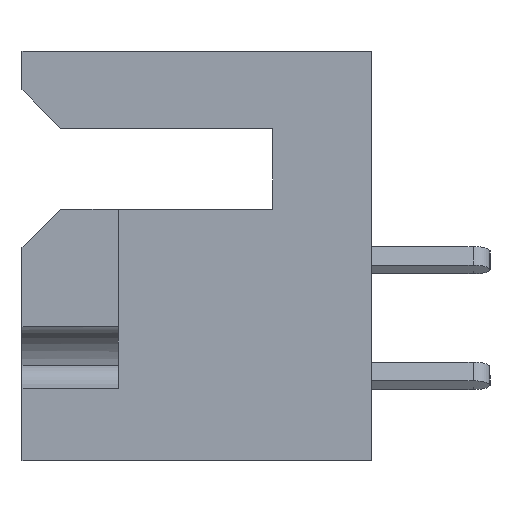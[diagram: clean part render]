
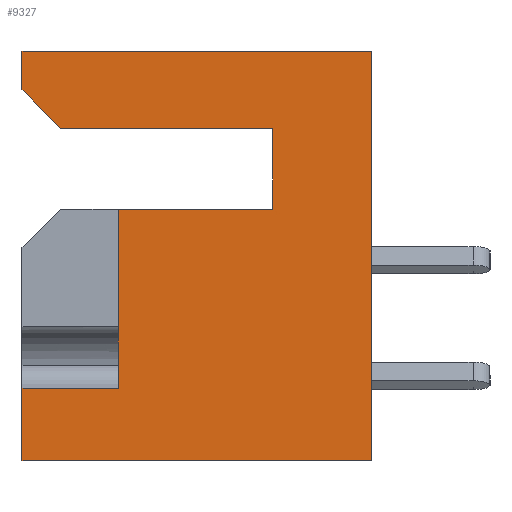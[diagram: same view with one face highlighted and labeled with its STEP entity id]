
A CAD part, left-side view. The second image highlights one B-rep face of the part: STEP entity #9327.
In plain terms, the highlighted planar face has unit normal (-1, 0, 0).
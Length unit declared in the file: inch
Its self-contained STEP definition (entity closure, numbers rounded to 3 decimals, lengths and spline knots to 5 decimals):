
#582 = DIRECTION ( 'NONE',  ( 0., 0., -1. ) ) ;
#656 = DIRECTION ( 'NONE',  ( 0., 0., 1. ) ) ;
#720 = EDGE_LOOP ( 'NONE', ( #2321, #5784, #2436, #14988, #20665, #20450, #15149, #14483, #7558, #4252, #10557 ) ) ;
#765 = VERTEX_POINT ( 'NONE', #15995 ) ;
#1047 = DIRECTION ( 'NONE',  ( 0., 0., 1. ) ) ;
#1205 = VECTOR ( 'NONE', #13760, 39.37008 ) ;
#1775 = CARTESIAN_POINT ( 'NONE',  ( 0., 0.128, -0.205 ) ) ;
#1846 = DIRECTION ( 'NONE',  ( 0., -1., 0. ) ) ;
#1978 = VERTEX_POINT ( 'NONE', #9057 ) ;
#2321 = ORIENTED_EDGE ( 'NONE', *, *, #4453, .T. ) ;
#2436 = ORIENTED_EDGE ( 'NONE', *, *, #13924, .T. ) ;
#2478 = CARTESIAN_POINT ( 'NONE',  ( 0., 0.453, -0.437 ) ) ;
#2807 = VERTEX_POINT ( 'NONE', #6285 ) ;
#3856 = VERTEX_POINT ( 'NONE', #13707 ) ;
#4141 = VECTOR ( 'NONE', #1846, 39.37008 ) ;
#4240 = VECTOR ( 'NONE', #19440, 39.37008 ) ;
#4252 = ORIENTED_EDGE ( 'NONE', *, *, #21017, .T. ) ;
#4259 = LINE ( 'NONE', #20620, #7377 ) ;
#4339 = EDGE_CURVE ( 'NONE', #19047, #16593, #14629, .T. ) ;
#4400 = EDGE_CURVE ( 'NONE', #15226, #4521, #13585, .T. ) ;
#4453 = EDGE_CURVE ( 'NONE', #1978, #4521, #5614, .T. ) ;
#4521 = VERTEX_POINT ( 'NONE', #2478 ) ;
#4609 = LINE ( 'NONE', #15171, #5126 ) ;
#4799 = DIRECTION ( 'NONE',  ( 0., -0.707, -0.707 ) ) ;
#5126 = VECTOR ( 'NONE', #18291, 39.37008 ) ;
#5201 = EDGE_CURVE ( 'NONE', #3856, #19978, #6075, .T. ) ;
#5295 = EDGE_CURVE ( 'NONE', #14636, #765, #8922, .T. ) ;
#5303 = DIRECTION ( 'NONE',  ( 0., 1., 0. ) ) ;
#5357 = DIRECTION ( 'NONE',  ( 0., 0., 1. ) ) ;
#5528 = CARTESIAN_POINT ( 'NONE',  ( 0., 0.128, -0.1 ) ) ;
#5614 = LINE ( 'NONE', #20326, #1205 ) ;
#5784 = ORIENTED_EDGE ( 'NONE', *, *, #4400, .F. ) ;
#6075 = LINE ( 'NONE', #15901, #11465 ) ;
#6285 = CARTESIAN_POINT ( 'NONE',  ( 0., 0.453, 0. ) ) ;
#6947 = LINE ( 'NONE', #1775, #15443 ) ;
#7377 = VECTOR ( 'NONE', #10815, 39.37008 ) ;
#7456 = PLANE ( 'NONE',  #13819 ) ;
#7558 = ORIENTED_EDGE ( 'NONE', *, *, #5201, .F. ) ;
#8922 = LINE ( 'NONE', #14588, #13541 ) ;
#9057 = CARTESIAN_POINT ( 'NONE',  ( 0., 0.328, -0.437 ) ) ;
#9215 = VECTOR ( 'NONE', #5357, 39.37008 ) ;
#9232 = CARTESIAN_POINT ( 'NONE',  ( 0., 0., -0.531 ) ) ;
#9327 = ADVANCED_FACE ( 'NONE', ( #21091 ), #7456, .F. ) ;
#10258 = CARTESIAN_POINT ( 'NONE',  ( 0., 0.328, -0.205 ) ) ;
#10482 = VERTEX_POINT ( 'NONE', #10258 ) ;
#10557 = ORIENTED_EDGE ( 'NONE', *, *, #10729, .F. ) ;
#10729 = EDGE_CURVE ( 'NONE', #1978, #10482, #4259, .T. ) ;
#10815 = DIRECTION ( 'NONE',  ( 0., 0., 1. ) ) ;
#11374 = EDGE_CURVE ( 'NONE', #14636, #2807, #14024, .T. ) ;
#11465 = VECTOR ( 'NONE', #1047, 39.37008 ) ;
#11797 = VECTOR ( 'NONE', #13655, 39.37008 ) ;
#11943 = CARTESIAN_POINT ( 'NONE',  ( 0., 0.453, 0. ) ) ;
#12940 = CARTESIAN_POINT ( 'NONE',  ( 0., 0.453, 0. ) ) ;
#13279 = CARTESIAN_POINT ( 'NONE',  ( 0., 0.453, -0.531 ) ) ;
#13541 = VECTOR ( 'NONE', #4799, 39.37008 ) ;
#13585 = LINE ( 'NONE', #11943, #20291 ) ;
#13655 = DIRECTION ( 'NONE',  ( 0., 1., 0. ) ) ;
#13707 = CARTESIAN_POINT ( 'NONE',  ( 0., 0.128, -0.205 ) ) ;
#13760 = DIRECTION ( 'NONE',  ( 0., 1., 0. ) ) ;
#13766 = CARTESIAN_POINT ( 'NONE',  ( 0., 0.453, -0.05 ) ) ;
#13819 = AXIS2_PLACEMENT_3D ( 'NONE', #20387, #17162, #582 ) ;
#13924 = EDGE_CURVE ( 'NONE', #15226, #19047, #15497, .T. ) ;
#14024 = LINE ( 'NONE', #12940, #4240 ) ;
#14483 = ORIENTED_EDGE ( 'NONE', *, *, #15991, .F. ) ;
#14588 = CARTESIAN_POINT ( 'NONE',  ( 0., 0.403, -0.1 ) ) ;
#14629 = LINE ( 'NONE', #18392, #9215 ) ;
#14636 = VERTEX_POINT ( 'NONE', #13766 ) ;
#14988 = ORIENTED_EDGE ( 'NONE', *, *, #4339, .T. ) ;
#15149 = ORIENTED_EDGE ( 'NONE', *, *, #5295, .T. ) ;
#15171 = CARTESIAN_POINT ( 'NONE',  ( 0., 0.453, 0. ) ) ;
#15226 = VERTEX_POINT ( 'NONE', #19521 ) ;
#15443 = VECTOR ( 'NONE', #5303, 39.37008 ) ;
#15497 = LINE ( 'NONE', #13279, #4141 ) ;
#15901 = CARTESIAN_POINT ( 'NONE',  ( 0., 0.128, -0.1 ) ) ;
#15991 = EDGE_CURVE ( 'NONE', #19978, #765, #17246, .T. ) ;
#15995 = CARTESIAN_POINT ( 'NONE',  ( 0., 0.403, -0.1 ) ) ;
#16593 = VERTEX_POINT ( 'NONE', #18966 ) ;
#17162 = DIRECTION ( 'NONE',  ( 1., 0., 0. ) ) ;
#17246 = LINE ( 'NONE', #5528, #11797 ) ;
#18291 = DIRECTION ( 'NONE',  ( 0., -1., 0. ) ) ;
#18356 = CARTESIAN_POINT ( 'NONE',  ( 0., 0.128, -0.1 ) ) ;
#18392 = CARTESIAN_POINT ( 'NONE',  ( 0., 0., 0. ) ) ;
#18966 = CARTESIAN_POINT ( 'NONE',  ( 0., 0., 0. ) ) ;
#19047 = VERTEX_POINT ( 'NONE', #9232 ) ;
#19440 = DIRECTION ( 'NONE',  ( 0., 0., 1. ) ) ;
#19521 = CARTESIAN_POINT ( 'NONE',  ( 0., 0.453, -0.531 ) ) ;
#19978 = VERTEX_POINT ( 'NONE', #18356 ) ;
#20291 = VECTOR ( 'NONE', #656, 39.37008 ) ;
#20326 = CARTESIAN_POINT ( 'NONE',  ( 0., 0.328, -0.437 ) ) ;
#20387 = CARTESIAN_POINT ( 'NONE',  ( 0., 0.453, 0. ) ) ;
#20450 = ORIENTED_EDGE ( 'NONE', *, *, #11374, .F. ) ;
#20620 = CARTESIAN_POINT ( 'NONE',  ( 0., 0.328, -0.205 ) ) ;
#20665 = ORIENTED_EDGE ( 'NONE', *, *, #20982, .F. ) ;
#20982 = EDGE_CURVE ( 'NONE', #2807, #16593, #4609, .T. ) ;
#21017 = EDGE_CURVE ( 'NONE', #3856, #10482, #6947, .T. ) ;
#21091 = FACE_OUTER_BOUND ( 'NONE', #720, .T. ) ;
